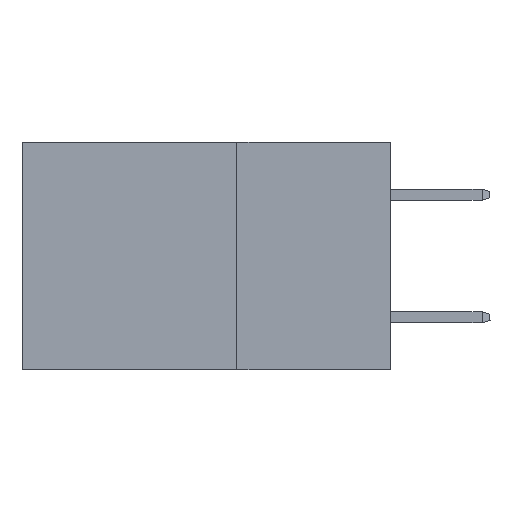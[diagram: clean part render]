
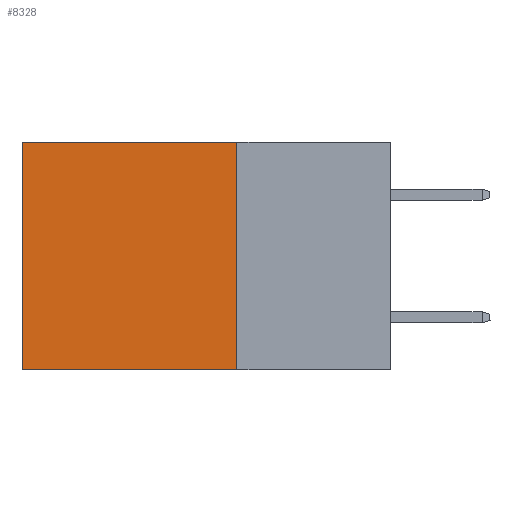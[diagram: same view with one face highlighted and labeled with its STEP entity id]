
A CAD part, left-side view. The second image highlights one B-rep face of the part: STEP entity #8328.
In plain terms, the highlighted planar face has unit normal (-1, 0, 0).
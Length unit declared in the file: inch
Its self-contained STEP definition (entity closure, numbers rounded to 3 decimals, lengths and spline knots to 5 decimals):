
#411 = EDGE_CURVE ( 'NONE', #21638, #30569, #28537, .T. ) ;
#946 = ORIENTED_EDGE ( 'NONE', *, *, #411, .T. ) ;
#1959 = ORIENTED_EDGE ( 'NONE', *, *, #11671, .F. ) ;
#3664 = CARTESIAN_POINT ( 'NONE',  ( 0.2875, 0.25, -0.37 ) ) ;
#3766 = CARTESIAN_POINT ( 'NONE',  ( 0.2875, 0.25, 0. ) ) ;
#4076 = DIRECTION ( 'NONE',  ( 0., 1., 0. ) ) ;
#4768 = VECTOR ( 'NONE', #4076, 39.37008 ) ;
#7020 = VERTEX_POINT ( 'NONE', #23207 ) ;
#7240 = CARTESIAN_POINT ( 'NONE',  ( 0.2875, 0.6, 0. ) ) ;
#7895 = DIRECTION ( 'NONE',  ( 0., 0., -1. ) ) ;
#8328 = ADVANCED_FACE ( 'NONE', ( #22299 ), #25908, .F. ) ;
#8707 = DIRECTION ( 'NONE',  ( 0., 1., 0. ) ) ;
#9240 = VERTEX_POINT ( 'NONE', #29692 ) ;
#9294 = LINE ( 'NONE', #3664, #4768 ) ;
#9436 = DIRECTION ( 'NONE',  ( 0., 0., -1. ) ) ;
#11616 = EDGE_LOOP ( 'NONE', ( #14102, #18158, #1959, #946 ) ) ;
#11671 = EDGE_CURVE ( 'NONE', #21638, #7020, #25347, .T. ) ;
#11954 = VECTOR ( 'NONE', #8707, 39.37008 ) ;
#12891 = DIRECTION ( 'NONE',  ( 0., 0., -1. ) ) ;
#13922 = DIRECTION ( 'NONE',  ( 1., 0., 0. ) ) ;
#14102 = ORIENTED_EDGE ( 'NONE', *, *, #14889, .T. ) ;
#14889 = EDGE_CURVE ( 'NONE', #30569, #9240, #23624, .T. ) ;
#16871 = VECTOR ( 'NONE', #12891, 39.37008 ) ;
#17649 = EDGE_CURVE ( 'NONE', #7020, #9240, #9294, .T. ) ;
#17888 = CARTESIAN_POINT ( 'NONE',  ( 0.2875, 0.25, 0. ) ) ;
#18134 = AXIS2_PLACEMENT_3D ( 'NONE', #18898, #13922, #9436 ) ;
#18158 = ORIENTED_EDGE ( 'NONE', *, *, #17649, .F. ) ;
#18898 = CARTESIAN_POINT ( 'NONE',  ( 0.2875, 0.25, 0. ) ) ;
#19486 = CARTESIAN_POINT ( 'NONE',  ( 0.2875, 0.25, 0. ) ) ;
#21638 = VERTEX_POINT ( 'NONE', #17888 ) ;
#22299 = FACE_OUTER_BOUND ( 'NONE', #11616, .T. ) ;
#23207 = CARTESIAN_POINT ( 'NONE',  ( 0.2875, 0.25, -0.37 ) ) ;
#23624 = LINE ( 'NONE', #27303, #16871 ) ;
#24972 = VECTOR ( 'NONE', #7895, 39.37008 ) ;
#25347 = LINE ( 'NONE', #19486, #24972 ) ;
#25908 = PLANE ( 'NONE',  #18134 ) ;
#27303 = CARTESIAN_POINT ( 'NONE',  ( 0.2875, 0.6, 0. ) ) ;
#28537 = LINE ( 'NONE', #3766, #11954 ) ;
#29692 = CARTESIAN_POINT ( 'NONE',  ( 0.2875, 0.6, -0.37 ) ) ;
#30569 = VERTEX_POINT ( 'NONE', #7240 ) ;
